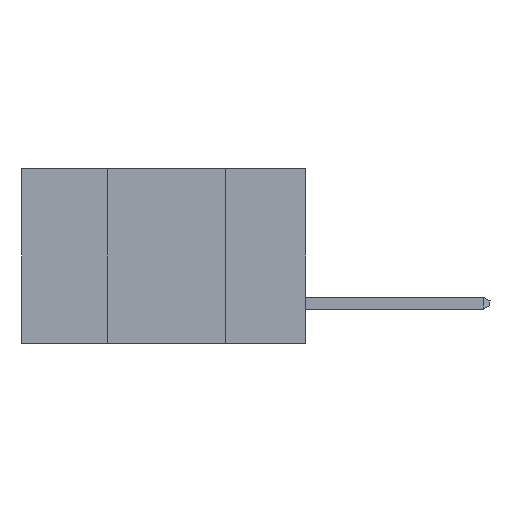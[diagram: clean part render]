
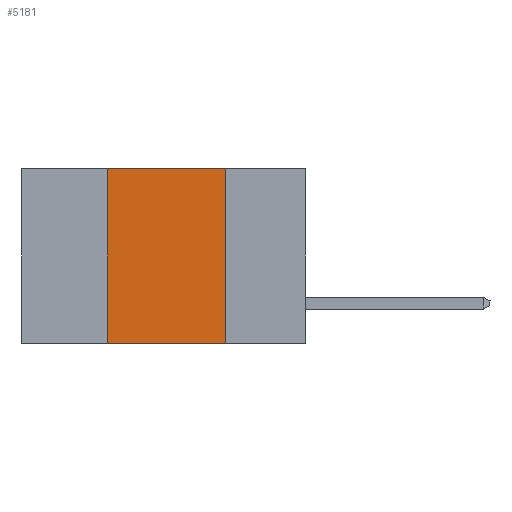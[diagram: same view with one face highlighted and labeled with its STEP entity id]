
A CAD part, left-side view. The second image highlights one B-rep face of the part: STEP entity #5181.
In plain terms, the highlighted planar face has unit normal (-1, 0, 0).
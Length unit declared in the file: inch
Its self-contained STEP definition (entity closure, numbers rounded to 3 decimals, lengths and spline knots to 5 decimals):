
#496 = CARTESIAN_POINT ( 'NONE',  ( 0., 0.6, -0.37 ) ) ;
#560 = VECTOR ( 'NONE', #4988, 39.37008 ) ;
#586 = EDGE_LOOP ( 'NONE', ( #11154, #3938, #9513, #11433 ) ) ;
#877 = EDGE_CURVE ( 'NONE', #8340, #4708, #18083, .T. ) ;
#1376 = DIRECTION ( 'NONE',  ( 0., -1., 0. ) ) ;
#1621 = CARTESIAN_POINT ( 'NONE',  ( 0., 0.6, 0. ) ) ;
#1646 = VECTOR ( 'NONE', #1376, 39.37008 ) ;
#3180 = CARTESIAN_POINT ( 'NONE',  ( 0., 0.42, -0.37 ) ) ;
#3332 = LINE ( 'NONE', #496, #560 ) ;
#3489 = EDGE_CURVE ( 'NONE', #6765, #8340, #7966, .T. ) ;
#3938 = ORIENTED_EDGE ( 'NONE', *, *, #877, .F. ) ;
#4111 = CARTESIAN_POINT ( 'NONE',  ( 0., 0.17, -0.37 ) ) ;
#4254 = EDGE_CURVE ( 'NONE', #6765, #13663, #3332, .T. ) ;
#4708 = VERTEX_POINT ( 'NONE', #13877 ) ;
#4750 = PLANE ( 'NONE',  #10136 ) ;
#4842 = DIRECTION ( 'NONE',  ( 0., 0., 1. ) ) ;
#4847 = DIRECTION ( 'NONE',  ( 1., 0., 0. ) ) ;
#4988 = DIRECTION ( 'NONE',  ( 0., -1., 0. ) ) ;
#5181 = ADVANCED_FACE ( 'NONE', ( #12200 ), #4750, .F. ) ;
#5586 = LINE ( 'NONE', #4111, #16749 ) ;
#6765 = VERTEX_POINT ( 'NONE', #9651 ) ;
#7121 = CARTESIAN_POINT ( 'NONE',  ( 0., 0.42, 0. ) ) ;
#7966 = LINE ( 'NONE', #3180, #11960 ) ;
#8340 = VERTEX_POINT ( 'NONE', #7121 ) ;
#9513 = ORIENTED_EDGE ( 'NONE', *, *, #3489, .F. ) ;
#9651 = CARTESIAN_POINT ( 'NONE',  ( 0., 0.42, -0.37 ) ) ;
#10136 = AXIS2_PLACEMENT_3D ( 'NONE', #1621, #4847, #16781 ) ;
#11154 = ORIENTED_EDGE ( 'NONE', *, *, #15104, .F. ) ;
#11433 = ORIENTED_EDGE ( 'NONE', *, *, #4254, .T. ) ;
#11960 = VECTOR ( 'NONE', #4842, 39.37008 ) ;
#12200 = FACE_OUTER_BOUND ( 'NONE', #586, .T. ) ;
#13440 = CARTESIAN_POINT ( 'NONE',  ( 0., 0.17, -0.37 ) ) ;
#13663 = VERTEX_POINT ( 'NONE', #13440 ) ;
#13877 = CARTESIAN_POINT ( 'NONE',  ( 0., 0.17, 0. ) ) ;
#15104 = EDGE_CURVE ( 'NONE', #4708, #13663, #5586, .T. ) ;
#15953 = DIRECTION ( 'NONE',  ( 0., 0., -1. ) ) ;
#16749 = VECTOR ( 'NONE', #15953, 39.37008 ) ;
#16781 = DIRECTION ( 'NONE',  ( 0., 0., -1. ) ) ;
#17883 = CARTESIAN_POINT ( 'NONE',  ( 0., 0.6, 0. ) ) ;
#18083 = LINE ( 'NONE', #17883, #1646 ) ;
